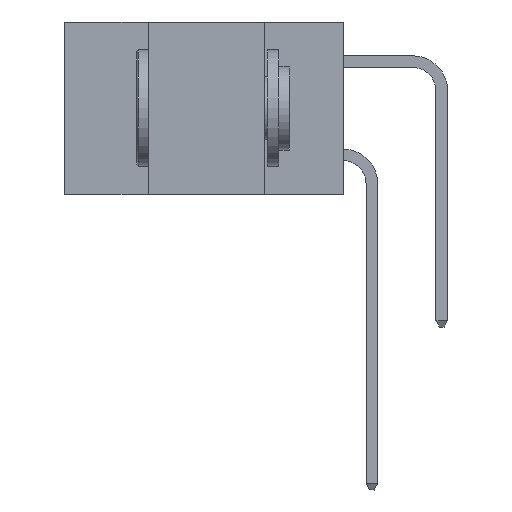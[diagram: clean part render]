
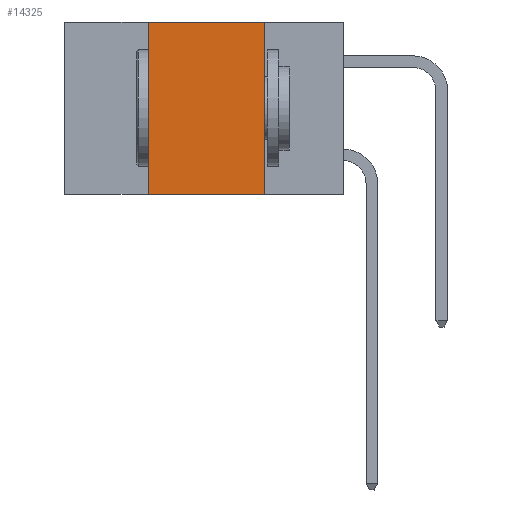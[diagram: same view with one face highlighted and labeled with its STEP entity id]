
A CAD part, left-side view. The second image highlights one B-rep face of the part: STEP entity #14325.
In plain terms, the highlighted planar face has unit normal (-1, 0, 0).
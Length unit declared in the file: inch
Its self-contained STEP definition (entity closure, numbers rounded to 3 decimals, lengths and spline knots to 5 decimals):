
#85 = VECTOR ( 'NONE', #12012, 39.37008 ) ;
#444 = DIRECTION ( 'NONE',  ( 1., 0., 0. ) ) ;
#1388 = ORIENTED_EDGE ( 'NONE', *, *, #14292, .F. ) ;
#1407 = ORIENTED_EDGE ( 'NONE', *, *, #8867, .F. ) ;
#1732 = ORIENTED_EDGE ( 'NONE', *, *, #3045, .F. ) ;
#1969 = ORIENTED_EDGE ( 'NONE', *, *, #5293, .T. ) ;
#3045 = EDGE_CURVE ( 'NONE', #9593, #4892, #3485, .T. ) ;
#3213 = EDGE_LOOP ( 'NONE', ( #1388, #1407, #1732, #1969 ) ) ;
#3485 = LINE ( 'NONE', #17779, #16362 ) ;
#4892 = VERTEX_POINT ( 'NONE', #20697 ) ;
#5293 = EDGE_CURVE ( 'NONE', #9593, #13200, #7618, .T. ) ;
#5822 = VERTEX_POINT ( 'NONE', #6948 ) ;
#6789 = AXIS2_PLACEMENT_3D ( 'NONE', #10515, #444, #12182 ) ;
#6948 = CARTESIAN_POINT ( 'NONE',  ( 0., 0.17, 0. ) ) ;
#7618 = LINE ( 'NONE', #14718, #11552 ) ;
#7931 = CARTESIAN_POINT ( 'NONE',  ( 0., 0.42, -0.37 ) ) ;
#8867 = EDGE_CURVE ( 'NONE', #4892, #5822, #13969, .T. ) ;
#9593 = VERTEX_POINT ( 'NONE', #7931 ) ;
#10479 = CARTESIAN_POINT ( 'NONE',  ( 0., 0.6, 0. ) ) ;
#10515 = CARTESIAN_POINT ( 'NONE',  ( 0., 0.6, 0. ) ) ;
#11552 = VECTOR ( 'NONE', #18004, 39.37008 ) ;
#12012 = DIRECTION ( 'NONE',  ( 0., -1., 0. ) ) ;
#12182 = DIRECTION ( 'NONE',  ( 0., 0., -1. ) ) ;
#13200 = VERTEX_POINT ( 'NONE', #20172 ) ;
#13722 = CARTESIAN_POINT ( 'NONE',  ( 0., 0.17, 0. ) ) ;
#13969 = LINE ( 'NONE', #10479, #85 ) ;
#14018 = VECTOR ( 'NONE', #20401, 39.37008 ) ;
#14292 = EDGE_CURVE ( 'NONE', #5822, #13200, #14556, .T. ) ;
#14325 = ADVANCED_FACE ( 'NONE', ( #17979 ), #20478, .F. ) ;
#14556 = LINE ( 'NONE', #13722, #14018 ) ;
#14718 = CARTESIAN_POINT ( 'NONE',  ( 0., 0.6, -0.37 ) ) ;
#16362 = VECTOR ( 'NONE', #19146, 39.37008 ) ;
#17779 = CARTESIAN_POINT ( 'NONE',  ( 0., 0.42, 0. ) ) ;
#17979 = FACE_OUTER_BOUND ( 'NONE', #3213, .T. ) ;
#18004 = DIRECTION ( 'NONE',  ( 0., -1., 0. ) ) ;
#19146 = DIRECTION ( 'NONE',  ( 0., 0., 1. ) ) ;
#20172 = CARTESIAN_POINT ( 'NONE',  ( 0., 0.17, -0.37 ) ) ;
#20401 = DIRECTION ( 'NONE',  ( 0., 0., -1. ) ) ;
#20478 = PLANE ( 'NONE',  #6789 ) ;
#20697 = CARTESIAN_POINT ( 'NONE',  ( 0., 0.42, 0. ) ) ;
